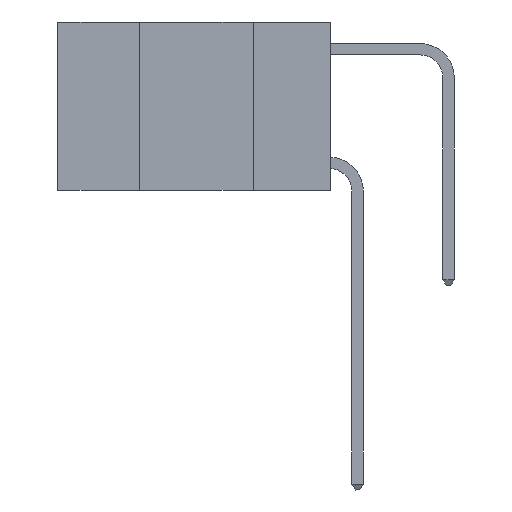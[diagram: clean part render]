
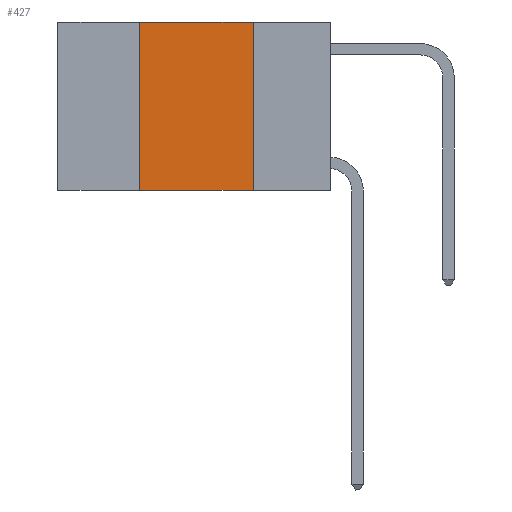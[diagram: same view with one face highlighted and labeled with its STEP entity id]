
A CAD part, left-side view. The second image highlights one B-rep face of the part: STEP entity #427.
In plain terms, the highlighted planar face has unit normal (-1, 0, 0).
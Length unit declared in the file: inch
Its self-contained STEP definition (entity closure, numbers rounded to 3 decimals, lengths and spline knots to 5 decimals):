
#321 = EDGE_CURVE ( 'NONE', #4563, #6627, #2023, .T. ) ;
#427 = ADVANCED_FACE ( 'NONE', ( #6203 ), #1549, .F. ) ;
#552 = CARTESIAN_POINT ( 'NONE',  ( 0., 0.6, 0. ) ) ;
#589 = CARTESIAN_POINT ( 'NONE',  ( 0., 0.6, -0.37 ) ) ;
#732 = EDGE_CURVE ( 'NONE', #7146, #6627, #9525, .T. ) ;
#1362 = ORIENTED_EDGE ( 'NONE', *, *, #321, .F. ) ;
#1549 = PLANE ( 'NONE',  #6260 ) ;
#1861 = EDGE_CURVE ( 'NONE', #7146, #9646, #3432, .T. ) ;
#2023 = LINE ( 'NONE', #4107, #7927 ) ;
#2633 = CARTESIAN_POINT ( 'NONE',  ( 0., 0.17, 0. ) ) ;
#2693 = CARTESIAN_POINT ( 'NONE',  ( 0., 0.6, 0. ) ) ;
#3022 = EDGE_CURVE ( 'NONE', #9646, #4563, #3658, .T. ) ;
#3432 = LINE ( 'NONE', #10172, #10474 ) ;
#3588 = ORIENTED_EDGE ( 'NONE', *, *, #3022, .F. ) ;
#3658 = LINE ( 'NONE', #552, #9711 ) ;
#3740 = DIRECTION ( 'NONE',  ( 0., -1., 0. ) ) ;
#3806 = CARTESIAN_POINT ( 'NONE',  ( 0., 0.42, 0. ) ) ;
#4107 = CARTESIAN_POINT ( 'NONE',  ( 0., 0.17, 0. ) ) ;
#4563 = VERTEX_POINT ( 'NONE', #2633 ) ;
#5100 = VECTOR ( 'NONE', #3740, 39.37008 ) ;
#5505 = DIRECTION ( 'NONE',  ( 0., -1., 0. ) ) ;
#5694 = ORIENTED_EDGE ( 'NONE', *, *, #1861, .F. ) ;
#5725 = CARTESIAN_POINT ( 'NONE',  ( 0., 0.17, -0.37 ) ) ;
#6203 = FACE_OUTER_BOUND ( 'NONE', #8717, .T. ) ;
#6260 = AXIS2_PLACEMENT_3D ( 'NONE', #2693, #8428, #6851 ) ;
#6627 = VERTEX_POINT ( 'NONE', #5725 ) ;
#6840 = DIRECTION ( 'NONE',  ( 0., 0., -1. ) ) ;
#6851 = DIRECTION ( 'NONE',  ( 0., 0., -1. ) ) ;
#7146 = VERTEX_POINT ( 'NONE', #7891 ) ;
#7789 = ORIENTED_EDGE ( 'NONE', *, *, #732, .T. ) ;
#7891 = CARTESIAN_POINT ( 'NONE',  ( 0., 0.42, -0.37 ) ) ;
#7927 = VECTOR ( 'NONE', #6840, 39.37008 ) ;
#8428 = DIRECTION ( 'NONE',  ( 1., 0., 0. ) ) ;
#8563 = DIRECTION ( 'NONE',  ( 0., 0., 1. ) ) ;
#8717 = EDGE_LOOP ( 'NONE', ( #1362, #3588, #5694, #7789 ) ) ;
#9525 = LINE ( 'NONE', #589, #5100 ) ;
#9646 = VERTEX_POINT ( 'NONE', #3806 ) ;
#9711 = VECTOR ( 'NONE', #5505, 39.37008 ) ;
#10172 = CARTESIAN_POINT ( 'NONE',  ( 0., 0.42, 0. ) ) ;
#10474 = VECTOR ( 'NONE', #8563, 39.37008 ) ;
